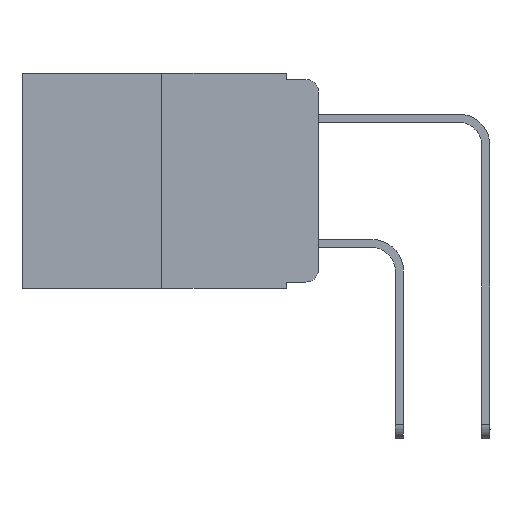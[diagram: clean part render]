
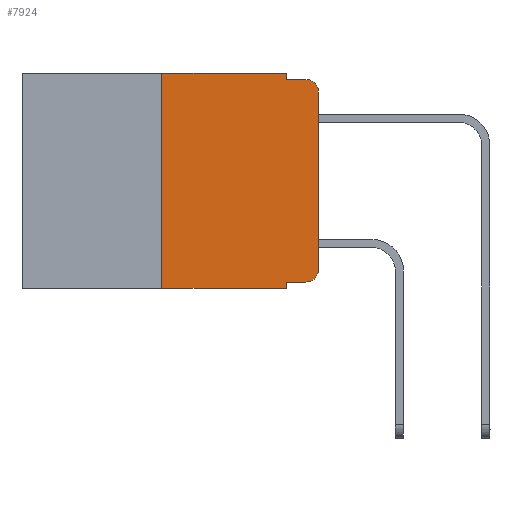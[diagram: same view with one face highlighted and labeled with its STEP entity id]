
A CAD part, left-side view. The second image highlights one B-rep face of the part: STEP entity #7924.
In plain terms, the highlighted planar face has unit normal (-1, 0, 0).
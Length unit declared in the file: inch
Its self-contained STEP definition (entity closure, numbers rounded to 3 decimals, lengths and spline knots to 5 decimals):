
#75 = VERTEX_POINT ( 'NONE', #5643 ) ;
#191 = VECTOR ( 'NONE', #15464, 39.37008 ) ;
#225 = VECTOR ( 'NONE', #19562, 39.37008 ) ;
#261 = CARTESIAN_POINT ( 'NONE',  ( 0., 0.02, -0.01 ) ) ;
#421 = CARTESIAN_POINT ( 'NONE',  ( 0., 0.02, -0.313 ) ) ;
#464 = VERTEX_POINT ( 'NONE', #6487 ) ;
#919 = FACE_OUTER_BOUND ( 'NONE', #9182, .T. ) ;
#1034 = VERTEX_POINT ( 'NONE', #11256 ) ;
#1063 = AXIS2_PLACEMENT_3D ( 'NONE', #19336, #6315, #21065 ) ;
#1882 = LINE ( 'NONE', #5194, #3135 ) ;
#1927 = DIRECTION ( 'NONE',  ( 0., -1., 0. ) ) ;
#2046 = CARTESIAN_POINT ( 'NONE',  ( 0., 0.473, 0. ) ) ;
#2091 = DIRECTION ( 'NONE',  ( 0., 0., -1. ) ) ;
#2788 = DIRECTION ( 'NONE',  ( 0., -1., 0. ) ) ;
#3135 = VECTOR ( 'NONE', #1927, 39.37008 ) ;
#3471 = EDGE_CURVE ( 'NONE', #5376, #1034, #5868, .T. ) ;
#3996 = DIRECTION ( 'NONE',  ( -1., 0., 0. ) ) ;
#4726 = LINE ( 'NONE', #10939, #12391 ) ;
#4806 = LINE ( 'NONE', #20357, #191 ) ;
#4893 = EDGE_CURVE ( 'NONE', #75, #6384, #6330, .T. ) ;
#5157 = VERTEX_POINT ( 'NONE', #18943 ) ;
#5194 = CARTESIAN_POINT ( 'NONE',  ( 0., 0.473, -0.343 ) ) ;
#5361 = EDGE_CURVE ( 'NONE', #5157, #13931, #18088, .T. ) ;
#5376 = VERTEX_POINT ( 'NONE', #6123 ) ;
#5643 = CARTESIAN_POINT ( 'NONE',  ( 0., 0.051, 0. ) ) ;
#5868 = LINE ( 'NONE', #17370, #20995 ) ;
#6123 = CARTESIAN_POINT ( 'NONE',  ( 0., 0.25, -0.343 ) ) ;
#6234 = VERTEX_POINT ( 'NONE', #261 ) ;
#6245 = EDGE_CURVE ( 'NONE', #5376, #8930, #1882, .T. ) ;
#6315 = DIRECTION ( 'NONE',  ( -1., 0., 0. ) ) ;
#6330 = LINE ( 'NONE', #8180, #225 ) ;
#6384 = VERTEX_POINT ( 'NONE', #7104 ) ;
#6487 = CARTESIAN_POINT ( 'NONE',  ( 0., 0.051, -0.333 ) ) ;
#6767 = CARTESIAN_POINT ( 'NONE',  ( 0., 0.051, -0.01 ) ) ;
#7104 = CARTESIAN_POINT ( 'NONE',  ( 0., 0.051, -0.01 ) ) ;
#7582 = ORIENTED_EDGE ( 'NONE', *, *, #12879, .T. ) ;
#7783 = CARTESIAN_POINT ( 'NONE',  ( 0., 0.051, -0.343 ) ) ;
#7924 = ADVANCED_FACE ( 'NONE', ( #919 ), #12089, .F. ) ;
#8055 = VERTEX_POINT ( 'NONE', #10755 ) ;
#8091 = ORIENTED_EDGE ( 'NONE', *, *, #18465, .F. ) ;
#8180 = CARTESIAN_POINT ( 'NONE',  ( 0., 0.051, 0. ) ) ;
#8343 = ORIENTED_EDGE ( 'NONE', *, *, #15564, .T. ) ;
#8502 = CIRCLE ( 'NONE', #1063, 0.02 ) ;
#8930 = VERTEX_POINT ( 'NONE', #7783 ) ;
#9182 = EDGE_LOOP ( 'NONE', ( #15735, #7582, #12970, #14016, #8091, #12797, #17640, #16918, #8343, #14835 ) ) ;
#10322 = EDGE_CURVE ( 'NONE', #8055, #5157, #20501, .T. ) ;
#10755 = CARTESIAN_POINT ( 'NONE',  ( 0., 0.02, -0.333 ) ) ;
#10939 = CARTESIAN_POINT ( 'NONE',  ( 0., 0.473, 0. ) ) ;
#11256 = CARTESIAN_POINT ( 'NONE',  ( 0., 0.25, 0. ) ) ;
#12089 = PLANE ( 'NONE',  #12765 ) ;
#12240 = DIRECTION ( 'NONE',  ( 0., 0., 1. ) ) ;
#12391 = VECTOR ( 'NONE', #2788, 39.37008 ) ;
#12765 = AXIS2_PLACEMENT_3D ( 'NONE', #2046, #17070, #13924 ) ;
#12797 = ORIENTED_EDGE ( 'NONE', *, *, #3471, .F. ) ;
#12879 = EDGE_CURVE ( 'NONE', #13931, #6234, #8502, .T. ) ;
#12970 = ORIENTED_EDGE ( 'NONE', *, *, #18824, .F. ) ;
#12988 = DIRECTION ( 'NONE',  ( 0., 0., 1. ) ) ;
#13602 = AXIS2_PLACEMENT_3D ( 'NONE', #421, #3996, #2091 ) ;
#13924 = DIRECTION ( 'NONE',  ( 0., 0., -1. ) ) ;
#13931 = VERTEX_POINT ( 'NONE', #19083 ) ;
#14016 = ORIENTED_EDGE ( 'NONE', *, *, #4893, .F. ) ;
#14481 = VECTOR ( 'NONE', #20441, 39.37008 ) ;
#14835 = ORIENTED_EDGE ( 'NONE', *, *, #10322, .T. ) ;
#15464 = DIRECTION ( 'NONE',  ( 0., 0., -1. ) ) ;
#15564 = EDGE_CURVE ( 'NONE', #464, #8055, #16562, .T. ) ;
#15735 = ORIENTED_EDGE ( 'NONE', *, *, #5361, .T. ) ;
#15967 = CARTESIAN_POINT ( 'NONE',  ( 0., 0., 0. ) ) ;
#16124 = EDGE_CURVE ( 'NONE', #464, #8930, #4806, .T. ) ;
#16562 = LINE ( 'NONE', #17003, #14481 ) ;
#16708 = VECTOR ( 'NONE', #18406, 39.37008 ) ;
#16918 = ORIENTED_EDGE ( 'NONE', *, *, #16124, .F. ) ;
#17003 = CARTESIAN_POINT ( 'NONE',  ( 0., 0.051, -0.333 ) ) ;
#17070 = DIRECTION ( 'NONE',  ( 1., 0., 0. ) ) ;
#17370 = CARTESIAN_POINT ( 'NONE',  ( 0., 0.25, 0. ) ) ;
#17640 = ORIENTED_EDGE ( 'NONE', *, *, #6245, .T. ) ;
#18088 = LINE ( 'NONE', #15967, #19117 ) ;
#18406 = DIRECTION ( 'NONE',  ( 0., -1., 0. ) ) ;
#18465 = EDGE_CURVE ( 'NONE', #1034, #75, #4726, .T. ) ;
#18824 = EDGE_CURVE ( 'NONE', #6384, #6234, #19539, .T. ) ;
#18943 = CARTESIAN_POINT ( 'NONE',  ( 0., 0., -0.313 ) ) ;
#19083 = CARTESIAN_POINT ( 'NONE',  ( 0., 0., -0.03 ) ) ;
#19117 = VECTOR ( 'NONE', #12988, 39.37008 ) ;
#19336 = CARTESIAN_POINT ( 'NONE',  ( 0., 0.02, -0.03 ) ) ;
#19539 = LINE ( 'NONE', #6767, #16708 ) ;
#19562 = DIRECTION ( 'NONE',  ( 0., 0., -1. ) ) ;
#20357 = CARTESIAN_POINT ( 'NONE',  ( 0., 0.051, 0. ) ) ;
#20441 = DIRECTION ( 'NONE',  ( 0., -1., 0. ) ) ;
#20501 = CIRCLE ( 'NONE', #13602, 0.02 ) ;
#20995 = VECTOR ( 'NONE', #12240, 39.37008 ) ;
#21065 = DIRECTION ( 'NONE',  ( 0., 0., -1. ) ) ;
